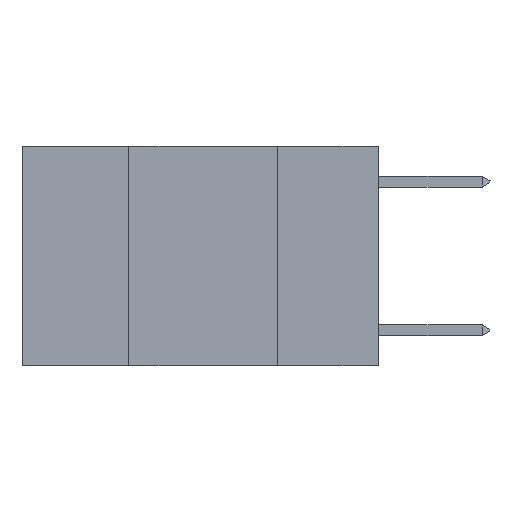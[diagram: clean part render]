
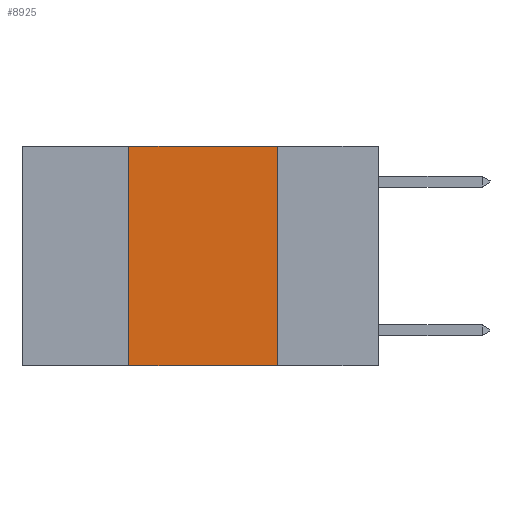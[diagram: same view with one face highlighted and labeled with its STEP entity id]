
A CAD part, left-side view. The second image highlights one B-rep face of the part: STEP entity #8925.
In plain terms, the highlighted planar face has unit normal (-1, 0, 0).
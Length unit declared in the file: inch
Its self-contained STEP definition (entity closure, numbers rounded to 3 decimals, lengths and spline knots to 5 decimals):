
#287 = VECTOR ( 'NONE', #2928, 39.37008 ) ;
#315 = CARTESIAN_POINT ( 'NONE',  ( 0., 0.17, 0. ) ) ;
#506 = LINE ( 'NONE', #8622, #4399 ) ;
#526 = ORIENTED_EDGE ( 'NONE', *, *, #4176, .T. ) ;
#699 = CARTESIAN_POINT ( 'NONE',  ( 0., 0.42, 0. ) ) ;
#804 = ORIENTED_EDGE ( 'NONE', *, *, #1856, .F. ) ;
#878 = DIRECTION ( 'NONE',  ( 1., 0., 0. ) ) ;
#960 = DIRECTION ( 'NONE',  ( 0., 0., -1. ) ) ;
#1036 = EDGE_CURVE ( 'NONE', #2793, #1228, #5286, .T. ) ;
#1164 = FACE_OUTER_BOUND ( 'NONE', #8482, .T. ) ;
#1228 = VERTEX_POINT ( 'NONE', #2596 ) ;
#1398 = LINE ( 'NONE', #4168, #6784 ) ;
#1818 = CARTESIAN_POINT ( 'NONE',  ( 0., 0.42, -0.37 ) ) ;
#1822 = EDGE_CURVE ( 'NONE', #7930, #2793, #1398, .T. ) ;
#1856 = EDGE_CURVE ( 'NONE', #4302, #7930, #6165, .T. ) ;
#2057 = CARTESIAN_POINT ( 'NONE',  ( 0., 0.42, 0. ) ) ;
#2596 = CARTESIAN_POINT ( 'NONE',  ( 0., 0.17, -0.37 ) ) ;
#2793 = VERTEX_POINT ( 'NONE', #8570 ) ;
#2928 = DIRECTION ( 'NONE',  ( 0., 0., 1. ) ) ;
#3061 = ORIENTED_EDGE ( 'NONE', *, *, #1036, .F. ) ;
#3299 = CARTESIAN_POINT ( 'NONE',  ( 0., 0.6, 0. ) ) ;
#3976 = DIRECTION ( 'NONE',  ( 0., -1., 0. ) ) ;
#4168 = CARTESIAN_POINT ( 'NONE',  ( 0., 0.6, 0. ) ) ;
#4176 = EDGE_CURVE ( 'NONE', #4302, #1228, #506, .T. ) ;
#4302 = VERTEX_POINT ( 'NONE', #1818 ) ;
#4399 = VECTOR ( 'NONE', #3976, 39.37008 ) ;
#5091 = VECTOR ( 'NONE', #960, 39.37008 ) ;
#5286 = LINE ( 'NONE', #315, #5091 ) ;
#5937 = PLANE ( 'NONE',  #7134 ) ;
#5962 = DIRECTION ( 'NONE',  ( 0., 0., -1. ) ) ;
#6135 = DIRECTION ( 'NONE',  ( 0., -1., 0. ) ) ;
#6165 = LINE ( 'NONE', #2057, #287 ) ;
#6784 = VECTOR ( 'NONE', #6135, 39.37008 ) ;
#7134 = AXIS2_PLACEMENT_3D ( 'NONE', #3299, #878, #5962 ) ;
#7930 = VERTEX_POINT ( 'NONE', #699 ) ;
#8095 = ORIENTED_EDGE ( 'NONE', *, *, #1822, .F. ) ;
#8482 = EDGE_LOOP ( 'NONE', ( #3061, #8095, #804, #526 ) ) ;
#8570 = CARTESIAN_POINT ( 'NONE',  ( 0., 0.17, 0. ) ) ;
#8622 = CARTESIAN_POINT ( 'NONE',  ( 0., 0.6, -0.37 ) ) ;
#8925 = ADVANCED_FACE ( 'NONE', ( #1164 ), #5937, .F. ) ;
